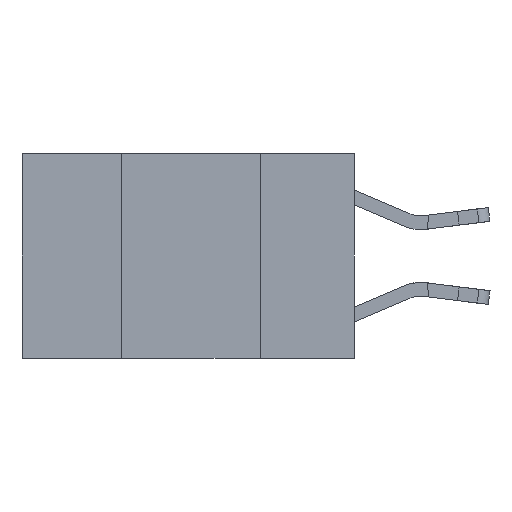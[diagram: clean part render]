
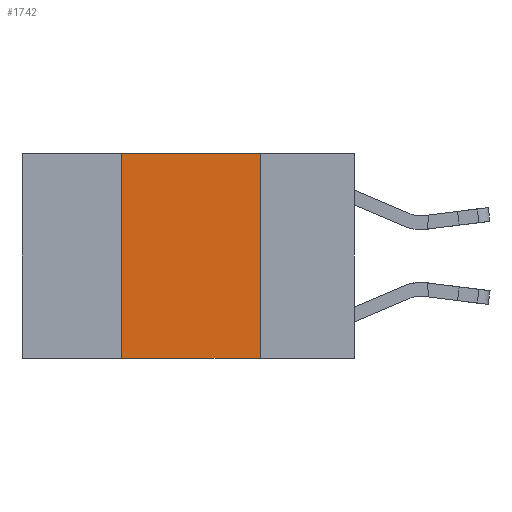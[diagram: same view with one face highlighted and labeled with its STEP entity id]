
A CAD part, left-side view. The second image highlights one B-rep face of the part: STEP entity #1742.
In plain terms, the highlighted planar face has unit normal (-1, 0, 0).
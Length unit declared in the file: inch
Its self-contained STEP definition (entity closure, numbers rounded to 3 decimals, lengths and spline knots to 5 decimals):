
#500 = DIRECTION ( 'NONE',  ( 0., -1., 0. ) ) ;
#922 = DIRECTION ( 'NONE',  ( 0., 0., -1. ) ) ;
#1158 = CARTESIAN_POINT ( 'NONE',  ( 0., 0.42, -0.37 ) ) ;
#1742 = ADVANCED_FACE ( 'NONE', ( #17100 ), #14717, .F. ) ;
#1903 = CARTESIAN_POINT ( 'NONE',  ( 0., 0.17, 0. ) ) ;
#2561 = DIRECTION ( 'NONE',  ( 0., -1., 0. ) ) ;
#2802 = EDGE_LOOP ( 'NONE', ( #27872, #23553, #11283, #8315 ) ) ;
#3061 = CARTESIAN_POINT ( 'NONE',  ( 0., 0.17, 0. ) ) ;
#5399 = CARTESIAN_POINT ( 'NONE',  ( 0., 0.6, 0. ) ) ;
#5442 = CARTESIAN_POINT ( 'NONE',  ( 0., 0.42, 0. ) ) ;
#6001 = VECTOR ( 'NONE', #2561, 39.37008 ) ;
#7619 = EDGE_CURVE ( 'NONE', #16169, #23336, #20666, .T. ) ;
#7751 = AXIS2_PLACEMENT_3D ( 'NONE', #25392, #15542, #24236 ) ;
#8315 = ORIENTED_EDGE ( 'NONE', *, *, #21538, .T. ) ;
#8752 = CARTESIAN_POINT ( 'NONE',  ( 0., 0.6, -0.37 ) ) ;
#10211 = EDGE_CURVE ( 'NONE', #25572, #26885, #26391, .T. ) ;
#11283 = ORIENTED_EDGE ( 'NONE', *, *, #10211, .F. ) ;
#11342 = DIRECTION ( 'NONE',  ( 0., 0., 1. ) ) ;
#11922 = CARTESIAN_POINT ( 'NONE',  ( 0., 0.42, 0. ) ) ;
#13485 = CARTESIAN_POINT ( 'NONE',  ( 0., 0.17, -0.37 ) ) ;
#14123 = VECTOR ( 'NONE', #500, 39.37008 ) ;
#14717 = PLANE ( 'NONE',  #7751 ) ;
#15542 = DIRECTION ( 'NONE',  ( 1., 0., 0. ) ) ;
#16169 = VERTEX_POINT ( 'NONE', #1903 ) ;
#17100 = FACE_OUTER_BOUND ( 'NONE', #2802, .T. ) ;
#18617 = VECTOR ( 'NONE', #922, 39.37008 ) ;
#20666 = LINE ( 'NONE', #3061, #18617 ) ;
#21538 = EDGE_CURVE ( 'NONE', #25572, #23336, #22219, .T. ) ;
#22219 = LINE ( 'NONE', #8752, #14123 ) ;
#23336 = VERTEX_POINT ( 'NONE', #13485 ) ;
#23553 = ORIENTED_EDGE ( 'NONE', *, *, #26040, .F. ) ;
#24236 = DIRECTION ( 'NONE',  ( 0., 0., -1. ) ) ;
#24512 = VECTOR ( 'NONE', #11342, 39.37008 ) ;
#24840 = LINE ( 'NONE', #5399, #6001 ) ;
#25392 = CARTESIAN_POINT ( 'NONE',  ( 0., 0.6, 0. ) ) ;
#25572 = VERTEX_POINT ( 'NONE', #1158 ) ;
#26040 = EDGE_CURVE ( 'NONE', #26885, #16169, #24840, .T. ) ;
#26391 = LINE ( 'NONE', #11922, #24512 ) ;
#26885 = VERTEX_POINT ( 'NONE', #5442 ) ;
#27872 = ORIENTED_EDGE ( 'NONE', *, *, #7619, .F. ) ;
